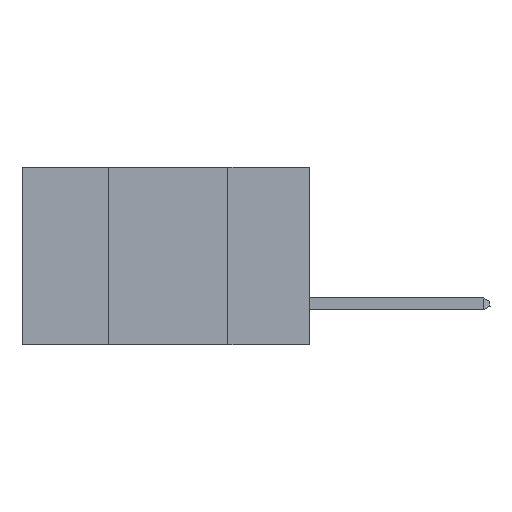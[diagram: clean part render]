
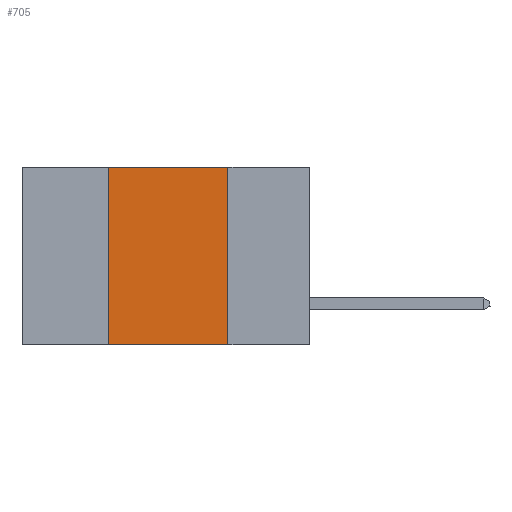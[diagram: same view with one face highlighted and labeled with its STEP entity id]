
A CAD part, left-side view. The second image highlights one B-rep face of the part: STEP entity #705.
In plain terms, the highlighted planar face has unit normal (-1, 0, 0).
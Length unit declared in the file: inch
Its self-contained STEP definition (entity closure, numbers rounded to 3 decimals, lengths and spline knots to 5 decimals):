
#705 = ADVANCED_FACE ( 'NONE', ( #8895 ), #6386, .F. ) ;
#800 = EDGE_CURVE ( 'NONE', #2096, #1382, #8530, .T. ) ;
#1101 = EDGE_CURVE ( 'NONE', #4346, #1382, #8642, .T. ) ;
#1382 = VERTEX_POINT ( 'NONE', #2323 ) ;
#1656 = CARTESIAN_POINT ( 'NONE',  ( 0., 0.6, -0.37 ) ) ;
#1709 = ORIENTED_EDGE ( 'NONE', *, *, #9950, .F. ) ;
#1730 = DIRECTION ( 'NONE',  ( 0., 0., -1. ) ) ;
#1757 = CARTESIAN_POINT ( 'NONE',  ( 0., 0.6, 0. ) ) ;
#2096 = VERTEX_POINT ( 'NONE', #6283 ) ;
#2099 = CARTESIAN_POINT ( 'NONE',  ( 0., 0.42, 0. ) ) ;
#2323 = CARTESIAN_POINT ( 'NONE',  ( 0., 0.17, -0.37 ) ) ;
#2453 = LINE ( 'NONE', #7678, #4769 ) ;
#2537 = ORIENTED_EDGE ( 'NONE', *, *, #800, .T. ) ;
#3656 = AXIS2_PLACEMENT_3D ( 'NONE', #1757, #7129, #1730 ) ;
#4002 = VECTOR ( 'NONE', #7578, 39.37008 ) ;
#4346 = VERTEX_POINT ( 'NONE', #6893 ) ;
#4581 = CARTESIAN_POINT ( 'NONE',  ( 0., 0.42, 0. ) ) ;
#4769 = VECTOR ( 'NONE', #8384, 39.37008 ) ;
#5410 = VERTEX_POINT ( 'NONE', #4581 ) ;
#6074 = VECTOR ( 'NONE', #6355, 39.37008 ) ;
#6113 = LINE ( 'NONE', #2099, #4002 ) ;
#6283 = CARTESIAN_POINT ( 'NONE',  ( 0., 0.42, -0.37 ) ) ;
#6355 = DIRECTION ( 'NONE',  ( 0., -1., 0. ) ) ;
#6386 = PLANE ( 'NONE',  #3656 ) ;
#6723 = DIRECTION ( 'NONE',  ( 0., 0., -1. ) ) ;
#6893 = CARTESIAN_POINT ( 'NONE',  ( 0., 0.17, 0. ) ) ;
#7077 = ORIENTED_EDGE ( 'NONE', *, *, #1101, .F. ) ;
#7129 = DIRECTION ( 'NONE',  ( 1., 0., 0. ) ) ;
#7578 = DIRECTION ( 'NONE',  ( 0., 0., 1. ) ) ;
#7678 = CARTESIAN_POINT ( 'NONE',  ( 0., 0.6, 0. ) ) ;
#8384 = DIRECTION ( 'NONE',  ( 0., -1., 0. ) ) ;
#8521 = VECTOR ( 'NONE', #6723, 39.37008 ) ;
#8530 = LINE ( 'NONE', #1656, #6074 ) ;
#8629 = ORIENTED_EDGE ( 'NONE', *, *, #8679, .F. ) ;
#8642 = LINE ( 'NONE', #9843, #8521 ) ;
#8679 = EDGE_CURVE ( 'NONE', #5410, #4346, #2453, .T. ) ;
#8895 = FACE_OUTER_BOUND ( 'NONE', #9801, .T. ) ;
#9801 = EDGE_LOOP ( 'NONE', ( #7077, #8629, #1709, #2537 ) ) ;
#9843 = CARTESIAN_POINT ( 'NONE',  ( 0., 0.17, 0. ) ) ;
#9950 = EDGE_CURVE ( 'NONE', #2096, #5410, #6113, .T. ) ;
